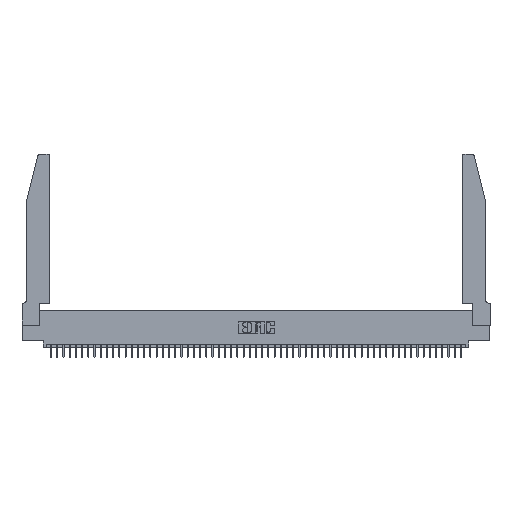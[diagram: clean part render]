
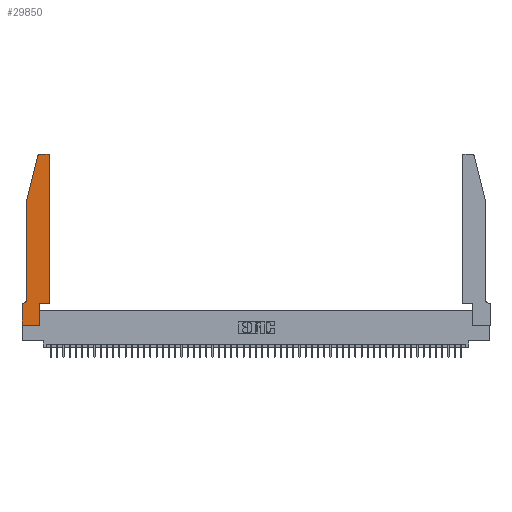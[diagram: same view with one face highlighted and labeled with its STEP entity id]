
A CAD part, top view. The second image highlights one B-rep face of the part: STEP entity #29850.
In plain terms, the highlighted planar face has unit normal (0, 0, 1).
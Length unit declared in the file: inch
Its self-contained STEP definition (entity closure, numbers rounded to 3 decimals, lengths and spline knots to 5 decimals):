
#446 = VERTEX_POINT ( 'NONE', #25836 ) ;
#746 = EDGE_CURVE ( 'NONE', #5519, #11976, #21402, .T. ) ;
#829 = VERTEX_POINT ( 'NONE', #44766 ) ;
#1539 = EDGE_CURVE ( 'NONE', #28907, #36410, #48158, .T. ) ;
#1970 = EDGE_CURVE ( 'NONE', #13250, #5519, #46783, .T. ) ;
#2245 = DIRECTION ( 'NONE',  ( -1., 0., 0. ) ) ;
#2844 = ORIENTED_EDGE ( 'NONE', *, *, #1539, .T. ) ;
#4929 = CARTESIAN_POINT ( 'NONE',  ( 0.4505, 2.72, 0.37 ) ) ;
#5136 = CARTESIAN_POINT ( 'NONE',  ( 0., 0.35, 0.37 ) ) ;
#5336 = EDGE_CURVE ( 'NONE', #446, #13250, #31450, .T. ) ;
#5519 = VERTEX_POINT ( 'NONE', #4929 ) ;
#5578 = EDGE_CURVE ( 'NONE', #18526, #50323, #9772, .T. ) ;
#7717 = CARTESIAN_POINT ( 'NONE',  ( 0.0755, 2., 0.37 ) ) ;
#7925 = EDGE_CURVE ( 'NONE', #53876, #829, #43430, .T. ) ;
#9191 = ORIENTED_EDGE ( 'NONE', *, *, #33299, .T. ) ;
#9293 = DIRECTION ( 'NONE',  ( 0., 0., -1. ) ) ;
#9344 = DIRECTION ( 'NONE',  ( 1., 0., 0. ) ) ;
#9436 = AXIS2_PLACEMENT_3D ( 'NONE', #19226, #48424, #23457 ) ;
#9772 = LINE ( 'NONE', #13561, #19627 ) ;
#10197 = CARTESIAN_POINT ( 'NONE',  ( 0., 0., 0.37 ) ) ;
#10511 = CARTESIAN_POINT ( 'NONE',  ( 0.25487, 2.72718, 0.37 ) ) ;
#11305 = VECTOR ( 'NONE', #17499, 39.37008 ) ;
#11367 = VECTOR ( 'NONE', #28582, 39.37008 ) ;
#11976 = VERTEX_POINT ( 'NONE', #27257 ) ;
#12635 = LINE ( 'NONE', #46501, #11305 ) ;
#13124 = CARTESIAN_POINT ( 'NONE',  ( 0.284, 2.72, 0.37 ) ) ;
#13250 = VERTEX_POINT ( 'NONE', #27454 ) ;
#13561 = CARTESIAN_POINT ( 'NONE',  ( 0., 0., 0.37 ) ) ;
#13704 = CARTESIAN_POINT ( 'NONE',  ( 0., 0.35, 0.37 ) ) ;
#13717 = LINE ( 'NONE', #23143, #34685 ) ;
#14266 = LINE ( 'NONE', #52942, #24084 ) ;
#16792 = DIRECTION ( 'NONE',  ( -1., 0., 0. ) ) ;
#17342 = DIRECTION ( 'NONE',  ( 1., 0., 0. ) ) ;
#17499 = DIRECTION ( 'NONE',  ( 0., -1., 0. ) ) ;
#17971 = ORIENTED_EDGE ( 'NONE', *, *, #746, .T. ) ;
#18468 = DIRECTION ( 'NONE',  ( 0., 1., 0. ) ) ;
#18526 = VERTEX_POINT ( 'NONE', #10197 ) ;
#19226 = CARTESIAN_POINT ( 'NONE',  ( 0.4205, 2.72, 0.37 ) ) ;
#19289 = LINE ( 'NONE', #47496, #40252 ) ;
#19627 = VECTOR ( 'NONE', #46965, 39.37008 ) ;
#20611 = EDGE_CURVE ( 'NONE', #50323, #446, #19289, .T. ) ;
#21402 = CIRCLE ( 'NONE', #9436, 0.03 ) ;
#21612 = AXIS2_PLACEMENT_3D ( 'NONE', #5136, #34478, #9344 ) ;
#21697 = ORIENTED_EDGE ( 'NONE', *, *, #20611, .T. ) ;
#23052 = ORIENTED_EDGE ( 'NONE', *, *, #47364, .T. ) ;
#23143 = CARTESIAN_POINT ( 'NONE',  ( 0.2605, 2.75, 0.37 ) ) ;
#23457 = DIRECTION ( 'NONE',  ( 1., 0., 0. ) ) ;
#24084 = VECTOR ( 'NONE', #40405, 39.37008 ) ;
#24214 = AXIS2_PLACEMENT_3D ( 'NONE', #13124, #42393, #17342 ) ;
#25836 = CARTESIAN_POINT ( 'NONE',  ( 0.2865, 0.35, 0.37 ) ) ;
#26889 = ORIENTED_EDGE ( 'NONE', *, *, #1970, .T. ) ;
#27221 = VERTEX_POINT ( 'NONE', #13704 ) ;
#27257 = CARTESIAN_POINT ( 'NONE',  ( 0.4205, 2.75, 0.37 ) ) ;
#27454 = CARTESIAN_POINT ( 'NONE',  ( 0.4505, 0.35, 0.37 ) ) ;
#28441 = DIRECTION ( 'NONE',  ( 0., 1., 0. ) ) ;
#28547 = ORIENTED_EDGE ( 'NONE', *, *, #5578, .T. ) ;
#28570 = ORIENTED_EDGE ( 'NONE', *, *, #44906, .T. ) ;
#28582 = DIRECTION ( 'NONE',  ( 0., -1., 0. ) ) ;
#28907 = VERTEX_POINT ( 'NONE', #49653 ) ;
#29850 = ADVANCED_FACE ( 'NONE', ( #39681 ), #30224, .T. ) ;
#30115 = VECTOR ( 'NONE', #45339, 39.37008 ) ;
#30224 = PLANE ( 'NONE',  #21612 ) ;
#31450 = LINE ( 'NONE', #32799, #30115 ) ;
#32799 = CARTESIAN_POINT ( 'NONE',  ( 0.4505, 0.35, 0.37 ) ) ;
#32961 = EDGE_CURVE ( 'NONE', #829, #42668, #42452, .T. ) ;
#33299 = EDGE_CURVE ( 'NONE', #36410, #53876, #14266, .T. ) ;
#34418 = CARTESIAN_POINT ( 'NONE',  ( 0.0055, 0.42, 0.37 ) ) ;
#34478 = DIRECTION ( 'NONE',  ( 0., 0., 1. ) ) ;
#34685 = VECTOR ( 'NONE', #2245, 39.37008 ) ;
#34948 = CARTESIAN_POINT ( 'NONE',  ( 0.0055, 0.35, 0.37 ) ) ;
#35764 = VECTOR ( 'NONE', #28441, 39.37008 ) ;
#36410 = VERTEX_POINT ( 'NONE', #10511 ) ;
#37654 = CARTESIAN_POINT ( 'NONE',  ( 0.0755, 0.35, 0.37 ) ) ;
#38306 = CARTESIAN_POINT ( 'NONE',  ( 0.0755, 2., 0.37 ) ) ;
#38621 = DIRECTION ( 'NONE',  ( -1., 0., 0. ) ) ;
#39681 = FACE_OUTER_BOUND ( 'NONE', #43684, .T. ) ;
#40252 = VECTOR ( 'NONE', #18468, 39.37008 ) ;
#40405 = DIRECTION ( 'NONE',  ( -0.239, -0.971, 0. ) ) ;
#40898 = CARTESIAN_POINT ( 'NONE',  ( 0.4505, 0.35, 0.37 ) ) ;
#42111 = CARTESIAN_POINT ( 'NONE',  ( 0.2865, 0., 0.37 ) ) ;
#42393 = DIRECTION ( 'NONE',  ( 0., 0., 1. ) ) ;
#42452 = CIRCLE ( 'NONE', #49662, 0.07 ) ;
#42668 = VERTEX_POINT ( 'NONE', #34948 ) ;
#43430 = LINE ( 'NONE', #7717, #11367 ) ;
#43473 = EDGE_CURVE ( 'NONE', #11976, #28907, #13717, .T. ) ;
#43684 = EDGE_LOOP ( 'NONE', ( #54111, #2844, #9191, #46033, #45902, #28570, #23052, #28547, #21697, #53557, #26889, #17971 ) ) ;
#44766 = CARTESIAN_POINT ( 'NONE',  ( 0.0755, 0.42, 0.37 ) ) ;
#44906 = EDGE_CURVE ( 'NONE', #42668, #27221, #52778, .T. ) ;
#45339 = DIRECTION ( 'NONE',  ( 1., 0., 0. ) ) ;
#45902 = ORIENTED_EDGE ( 'NONE', *, *, #32961, .T. ) ;
#46033 = ORIENTED_EDGE ( 'NONE', *, *, #7925, .T. ) ;
#46501 = CARTESIAN_POINT ( 'NONE',  ( 0., 0., 0.37 ) ) ;
#46783 = LINE ( 'NONE', #40898, #35764 ) ;
#46965 = DIRECTION ( 'NONE',  ( 1., 0., 0. ) ) ;
#47364 = EDGE_CURVE ( 'NONE', #27221, #18526, #12635, .T. ) ;
#47496 = CARTESIAN_POINT ( 'NONE',  ( 0.2865, 0.35, 0.37 ) ) ;
#48158 = CIRCLE ( 'NONE', #24214, 0.03 ) ;
#48424 = DIRECTION ( 'NONE',  ( 0., 0., 1. ) ) ;
#49653 = CARTESIAN_POINT ( 'NONE',  ( 0.284, 2.75, 0.37 ) ) ;
#49662 = AXIS2_PLACEMENT_3D ( 'NONE', #34418, #9293, #38621 ) ;
#50323 = VERTEX_POINT ( 'NONE', #42111 ) ;
#51454 = VECTOR ( 'NONE', #16792, 39.37008 ) ;
#52778 = LINE ( 'NONE', #37654, #51454 ) ;
#52942 = CARTESIAN_POINT ( 'NONE',  ( 0.0755, 2., 0.37 ) ) ;
#53557 = ORIENTED_EDGE ( 'NONE', *, *, #5336, .T. ) ;
#53876 = VERTEX_POINT ( 'NONE', #38306 ) ;
#54111 = ORIENTED_EDGE ( 'NONE', *, *, #43473, .T. ) ;
